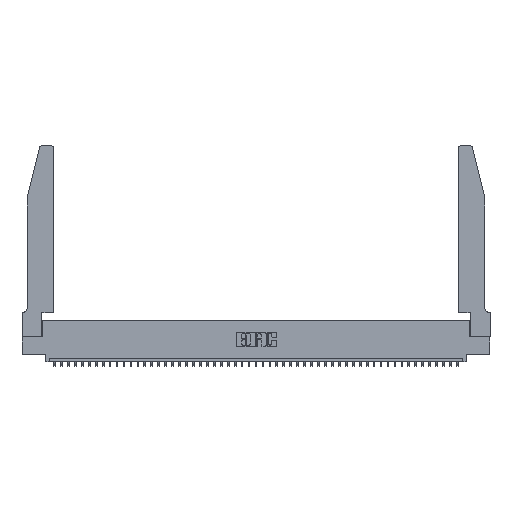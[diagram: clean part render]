
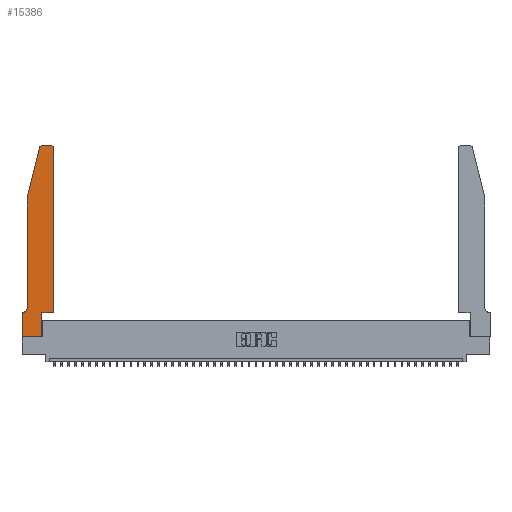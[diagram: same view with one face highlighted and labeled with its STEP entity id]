
A CAD part, top view. The second image highlights one B-rep face of the part: STEP entity #15386.
In plain terms, the highlighted planar face has unit normal (0, 0, 1).
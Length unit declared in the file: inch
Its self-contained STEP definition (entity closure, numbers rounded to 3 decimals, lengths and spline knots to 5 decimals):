
#1468 = CARTESIAN_POINT ( 'NONE',  ( 0.284, 2.72, 0.37 ) ) ;
#1873 = ORIENTED_EDGE ( 'NONE', *, *, #9807, .T. ) ;
#1919 = EDGE_CURVE ( 'NONE', #16530, #44441, #17550, .T. ) ;
#2003 = VECTOR ( 'NONE', #4671, 39.37008 ) ;
#2202 = CIRCLE ( 'NONE', #8358, 0.07 ) ;
#3143 = ORIENTED_EDGE ( 'NONE', *, *, #18166, .T. ) ;
#3317 = DIRECTION ( 'NONE',  ( 0., 0., -1. ) ) ;
#3567 = ORIENTED_EDGE ( 'NONE', *, *, #6218, .T. ) ;
#3688 = EDGE_CURVE ( 'NONE', #45173, #12233, #45188, .T. ) ;
#4066 = AXIS2_PLACEMENT_3D ( 'NONE', #43284, #7447, #7606 ) ;
#4671 = DIRECTION ( 'NONE',  ( -0.239, -0.971, 0. ) ) ;
#5535 = ORIENTED_EDGE ( 'NONE', *, *, #44376, .T. ) ;
#5974 = DIRECTION ( 'NONE',  ( 0., 0., 1. ) ) ;
#6012 = CARTESIAN_POINT ( 'NONE',  ( 0.25487, 2.72718, 0.37 ) ) ;
#6133 = PLANE ( 'NONE',  #43425 ) ;
#6218 = EDGE_CURVE ( 'NONE', #8654, #43536, #2202, .T. ) ;
#6481 = CARTESIAN_POINT ( 'NONE',  ( 0., 0., 0.37 ) ) ;
#6707 = LINE ( 'NONE', #8854, #10128 ) ;
#6850 = DIRECTION ( 'NONE',  ( 1., 0., 0. ) ) ;
#7447 = DIRECTION ( 'NONE',  ( 0., 0., 1. ) ) ;
#7606 = DIRECTION ( 'NONE',  ( 1., 0., 0. ) ) ;
#7725 = EDGE_CURVE ( 'NONE', #20229, #8654, #46583, .T. ) ;
#8358 = AXIS2_PLACEMENT_3D ( 'NONE', #25147, #3317, #17653 ) ;
#8654 = VERTEX_POINT ( 'NONE', #41051 ) ;
#8854 = CARTESIAN_POINT ( 'NONE',  ( 0.2865, 0.35, 0.37 ) ) ;
#9298 = CARTESIAN_POINT ( 'NONE',  ( 0., 0.35, 0.37 ) ) ;
#9759 = EDGE_CURVE ( 'NONE', #12233, #17185, #36189, .T. ) ;
#9807 = EDGE_CURVE ( 'NONE', #42559, #20229, #44704, .T. ) ;
#10071 = DIRECTION ( 'NONE',  ( -1., 0., 0. ) ) ;
#10128 = VECTOR ( 'NONE', #23706, 39.37008 ) ;
#10219 = FACE_OUTER_BOUND ( 'NONE', #40117, .T. ) ;
#11333 = ORIENTED_EDGE ( 'NONE', *, *, #9759, .T. ) ;
#12233 = VERTEX_POINT ( 'NONE', #35836 ) ;
#12258 = VERTEX_POINT ( 'NONE', #17359 ) ;
#12284 = DIRECTION ( 'NONE',  ( -1., 0., 0. ) ) ;
#12550 = ORIENTED_EDGE ( 'NONE', *, *, #3688, .T. ) ;
#12581 = CARTESIAN_POINT ( 'NONE',  ( 0.284, 2.75, 0.37 ) ) ;
#12955 = CARTESIAN_POINT ( 'NONE',  ( 0.0755, 2., 0.37 ) ) ;
#13856 = CARTESIAN_POINT ( 'NONE',  ( 0.4505, 0.35, 0.37 ) ) ;
#14614 = CARTESIAN_POINT ( 'NONE',  ( 0.0755, 2., 0.37 ) ) ;
#14918 = DIRECTION ( 'NONE',  ( 0., -1., 0. ) ) ;
#15386 = ADVANCED_FACE ( 'NONE', ( #10219 ), #6133, .T. ) ;
#15497 = CARTESIAN_POINT ( 'NONE',  ( 0.0755, 2., 0.37 ) ) ;
#16530 = VERTEX_POINT ( 'NONE', #38443 ) ;
#16623 = ORIENTED_EDGE ( 'NONE', *, *, #1919, .T. ) ;
#17185 = VERTEX_POINT ( 'NONE', #12581 ) ;
#17188 = EDGE_CURVE ( 'NONE', #17185, #42559, #26621, .T. ) ;
#17359 = CARTESIAN_POINT ( 'NONE',  ( 0.2865, 0.35, 0.37 ) ) ;
#17550 = LINE ( 'NONE', #22565, #38601 ) ;
#17653 = DIRECTION ( 'NONE',  ( -1., 0., 0. ) ) ;
#18166 = EDGE_CURVE ( 'NONE', #28678, #45173, #26591, .T. ) ;
#19720 = AXIS2_PLACEMENT_3D ( 'NONE', #1468, #20099, #23607 ) ;
#20099 = DIRECTION ( 'NONE',  ( 0., 0., 1. ) ) ;
#20229 = VERTEX_POINT ( 'NONE', #14614 ) ;
#20533 = VECTOR ( 'NONE', #10071, 39.37008 ) ;
#22016 = VECTOR ( 'NONE', #40666, 39.37008 ) ;
#22565 = CARTESIAN_POINT ( 'NONE',  ( 0., 0., 0.37 ) ) ;
#22721 = VECTOR ( 'NONE', #6850, 39.37008 ) ;
#23075 = CARTESIAN_POINT ( 'NONE',  ( 0., 0., 0.37 ) ) ;
#23607 = DIRECTION ( 'NONE',  ( 1., 0., 0. ) ) ;
#23655 = ORIENTED_EDGE ( 'NONE', *, *, #27491, .T. ) ;
#23706 = DIRECTION ( 'NONE',  ( 0., 1., 0. ) ) ;
#24286 = CARTESIAN_POINT ( 'NONE',  ( 0.2865, 0., 0.37 ) ) ;
#25147 = CARTESIAN_POINT ( 'NONE',  ( 0.0055, 0.42, 0.37 ) ) ;
#25737 = CARTESIAN_POINT ( 'NONE',  ( 0.4505, 2.72, 0.37 ) ) ;
#26028 = ORIENTED_EDGE ( 'NONE', *, *, #7725, .T. ) ;
#26535 = VECTOR ( 'NONE', #12284, 39.37008 ) ;
#26591 = LINE ( 'NONE', #33064, #22016 ) ;
#26621 = CIRCLE ( 'NONE', #19720, 0.03 ) ;
#27280 = VECTOR ( 'NONE', #44989, 39.37008 ) ;
#27491 = EDGE_CURVE ( 'NONE', #44441, #43370, #46566, .T. ) ;
#28678 = VERTEX_POINT ( 'NONE', #44426 ) ;
#29003 = LINE ( 'NONE', #13856, #22721 ) ;
#32540 = CARTESIAN_POINT ( 'NONE',  ( 0.0755, 0.35, 0.37 ) ) ;
#33004 = CARTESIAN_POINT ( 'NONE',  ( 0.0055, 0.35, 0.37 ) ) ;
#33064 = CARTESIAN_POINT ( 'NONE',  ( 0.4505, 0.35, 0.37 ) ) ;
#34630 = DIRECTION ( 'NONE',  ( 1., 0., 0. ) ) ;
#35836 = CARTESIAN_POINT ( 'NONE',  ( 0.4205, 2.75, 0.37 ) ) ;
#36189 = LINE ( 'NONE', #40003, #26535 ) ;
#36794 = ORIENTED_EDGE ( 'NONE', *, *, #43490, .T. ) ;
#36850 = ORIENTED_EDGE ( 'NONE', *, *, #17188, .T. ) ;
#38125 = LINE ( 'NONE', #32540, #20533 ) ;
#38443 = CARTESIAN_POINT ( 'NONE',  ( 0., 0.35, 0.37 ) ) ;
#38601 = VECTOR ( 'NONE', #14918, 39.37008 ) ;
#39224 = VECTOR ( 'NONE', #42098, 39.37008 ) ;
#40003 = CARTESIAN_POINT ( 'NONE',  ( 0.2605, 2.75, 0.37 ) ) ;
#40117 = EDGE_LOOP ( 'NONE', ( #11333, #36850, #1873, #26028, #3567, #36794, #16623, #23655, #5535, #47024, #3143, #12550 ) ) ;
#40666 = DIRECTION ( 'NONE',  ( 0., 1., 0. ) ) ;
#41051 = CARTESIAN_POINT ( 'NONE',  ( 0.0755, 0.42, 0.37 ) ) ;
#42098 = DIRECTION ( 'NONE',  ( 0., -1., 0. ) ) ;
#42559 = VERTEX_POINT ( 'NONE', #6012 ) ;
#43284 = CARTESIAN_POINT ( 'NONE',  ( 0.4205, 2.72, 0.37 ) ) ;
#43370 = VERTEX_POINT ( 'NONE', #24286 ) ;
#43425 = AXIS2_PLACEMENT_3D ( 'NONE', #9298, #5974, #34630 ) ;
#43490 = EDGE_CURVE ( 'NONE', #43536, #16530, #38125, .T. ) ;
#43536 = VERTEX_POINT ( 'NONE', #33004 ) ;
#43999 = EDGE_CURVE ( 'NONE', #12258, #28678, #29003, .T. ) ;
#44376 = EDGE_CURVE ( 'NONE', #43370, #12258, #6707, .T. ) ;
#44426 = CARTESIAN_POINT ( 'NONE',  ( 0.4505, 0.35, 0.37 ) ) ;
#44441 = VERTEX_POINT ( 'NONE', #6481 ) ;
#44704 = LINE ( 'NONE', #15497, #2003 ) ;
#44989 = DIRECTION ( 'NONE',  ( 1., 0., 0. ) ) ;
#45173 = VERTEX_POINT ( 'NONE', #25737 ) ;
#45188 = CIRCLE ( 'NONE', #4066, 0.03 ) ;
#46566 = LINE ( 'NONE', #23075, #27280 ) ;
#46583 = LINE ( 'NONE', #12955, #39224 ) ;
#47024 = ORIENTED_EDGE ( 'NONE', *, *, #43999, .T. ) ;
